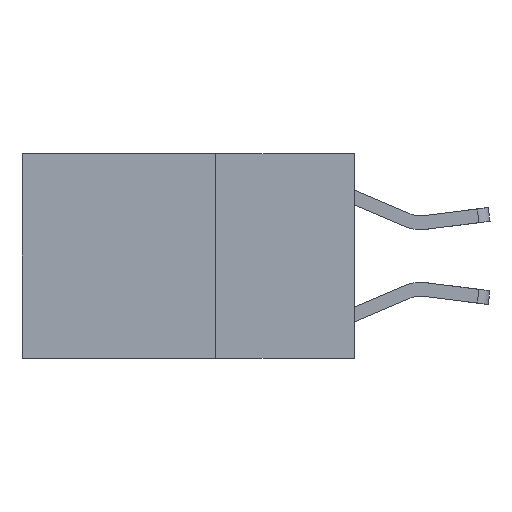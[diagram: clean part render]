
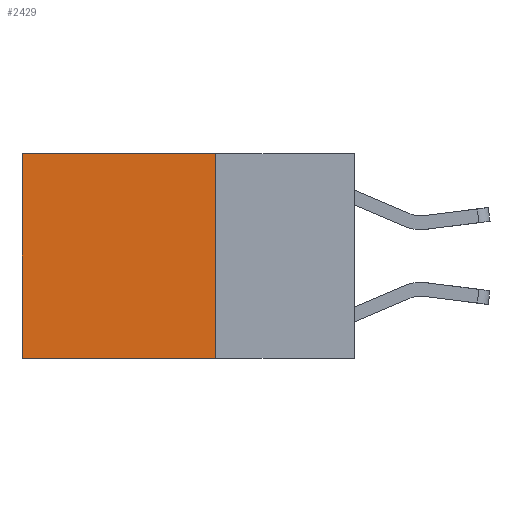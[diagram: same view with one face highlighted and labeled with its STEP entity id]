
A CAD part, left-side view. The second image highlights one B-rep face of the part: STEP entity #2429.
In plain terms, the highlighted planar face has unit normal (-1, 0, 0).
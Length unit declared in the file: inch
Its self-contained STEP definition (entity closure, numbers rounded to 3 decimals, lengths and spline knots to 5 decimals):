
#52 = LINE ( 'NONE', #6386, #8134 ) ;
#76 = DIRECTION ( 'NONE',  ( 0., 0., -1. ) ) ;
#89 = DIRECTION ( 'NONE',  ( 0., 0., -1. ) ) ;
#775 = PLANE ( 'NONE',  #4699 ) ;
#879 = CARTESIAN_POINT ( 'NONE',  ( 0.2625, 0.25, 0. ) ) ;
#1078 = LINE ( 'NONE', #879, #9267 ) ;
#1141 = EDGE_CURVE ( 'NONE', #3494, #8711, #52, .T. ) ;
#1726 = EDGE_CURVE ( 'NONE', #3494, #8490, #1078, .T. ) ;
#1828 = EDGE_CURVE ( 'NONE', #8711, #4868, #9353, .T. ) ;
#1970 = CARTESIAN_POINT ( 'NONE',  ( 0.2625, 0.6, -0.37 ) ) ;
#2049 = EDGE_CURVE ( 'NONE', #8490, #4868, #8109, .T. ) ;
#2429 = ADVANCED_FACE ( 'NONE', ( #3834 ), #775, .F. ) ;
#2435 = CARTESIAN_POINT ( 'NONE',  ( 0.2625, 0.25, 0. ) ) ;
#2941 = EDGE_LOOP ( 'NONE', ( #8305, #8660, #8667, #8586 ) ) ;
#3494 = VERTEX_POINT ( 'NONE', #7835 ) ;
#3817 = CARTESIAN_POINT ( 'NONE',  ( 0.2625, 0.25, -0.37 ) ) ;
#3834 = FACE_OUTER_BOUND ( 'NONE', #2941, .T. ) ;
#4162 = DIRECTION ( 'NONE',  ( 1., 0., 0. ) ) ;
#4699 = AXIS2_PLACEMENT_3D ( 'NONE', #2435, #4162, #4983 ) ;
#4868 = VERTEX_POINT ( 'NONE', #1970 ) ;
#4914 = CARTESIAN_POINT ( 'NONE',  ( 0.2625, 0.6, 0. ) ) ;
#4983 = DIRECTION ( 'NONE',  ( 0., 0., -1. ) ) ;
#5268 = DIRECTION ( 'NONE',  ( 0., 1., 0. ) ) ;
#5531 = VECTOR ( 'NONE', #89, 39.37008 ) ;
#5904 = VECTOR ( 'NONE', #5268, 39.37008 ) ;
#6265 = DIRECTION ( 'NONE',  ( 0., 1., 0. ) ) ;
#6386 = CARTESIAN_POINT ( 'NONE',  ( 0.2625, 0.25, 0. ) ) ;
#7188 = CARTESIAN_POINT ( 'NONE',  ( 0.2625, 0.6, 0. ) ) ;
#7677 = CARTESIAN_POINT ( 'NONE',  ( 0.2625, 0.25, -0.37 ) ) ;
#7835 = CARTESIAN_POINT ( 'NONE',  ( 0.2625, 0.25, 0. ) ) ;
#8109 = LINE ( 'NONE', #3817, #5904 ) ;
#8134 = VECTOR ( 'NONE', #6265, 39.37008 ) ;
#8305 = ORIENTED_EDGE ( 'NONE', *, *, #1828, .T. ) ;
#8490 = VERTEX_POINT ( 'NONE', #7677 ) ;
#8586 = ORIENTED_EDGE ( 'NONE', *, *, #1141, .T. ) ;
#8660 = ORIENTED_EDGE ( 'NONE', *, *, #2049, .F. ) ;
#8667 = ORIENTED_EDGE ( 'NONE', *, *, #1726, .F. ) ;
#8711 = VERTEX_POINT ( 'NONE', #4914 ) ;
#9267 = VECTOR ( 'NONE', #76, 39.37008 ) ;
#9353 = LINE ( 'NONE', #7188, #5531 ) ;
